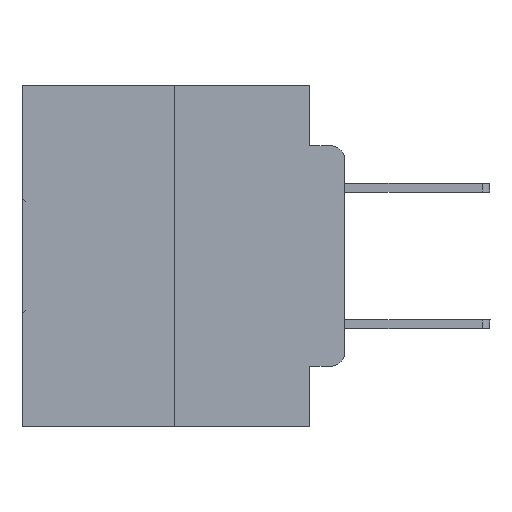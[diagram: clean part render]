
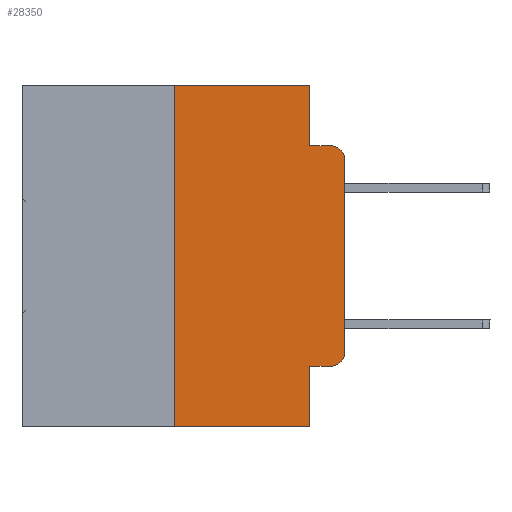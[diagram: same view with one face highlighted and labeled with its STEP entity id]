
A CAD part, left-side view. The second image highlights one B-rep face of the part: STEP entity #28350.
In plain terms, the highlighted planar face has unit normal (-1, 0, 0).
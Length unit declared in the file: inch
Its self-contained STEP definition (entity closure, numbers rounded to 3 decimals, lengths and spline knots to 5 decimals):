
#90 = CIRCLE ( 'NONE', #5570, 0.02 ) ;
#978 = CARTESIAN_POINT ( 'NONE',  ( 0., 0.25, 0. ) ) ;
#1286 = VECTOR ( 'NONE', #7229, 39.37008 ) ;
#1946 = CARTESIAN_POINT ( 'NONE',  ( 0., 0.25, -0.5 ) ) ;
#2361 = EDGE_CURVE ( 'NONE', #21545, #8161, #90, .T. ) ;
#2378 = VERTEX_POINT ( 'NONE', #16070 ) ;
#3023 = DIRECTION ( 'NONE',  ( -1., 0., 0. ) ) ;
#3044 = LINE ( 'NONE', #3188, #24980 ) ;
#3188 = CARTESIAN_POINT ( 'NONE',  ( 0., 0.25, 0. ) ) ;
#3230 = EDGE_CURVE ( 'NONE', #10841, #24574, #9522, .T. ) ;
#4170 = CARTESIAN_POINT ( 'NONE',  ( 0., 0.051, -0.0885 ) ) ;
#4710 = ORIENTED_EDGE ( 'NONE', *, *, #30780, .F. ) ;
#4950 = DIRECTION ( 'NONE',  ( 0., -1., 0. ) ) ;
#5284 = CARTESIAN_POINT ( 'NONE',  ( 0., 0.051, 0. ) ) ;
#5570 = AXIS2_PLACEMENT_3D ( 'NONE', #30448, #3023, #27502 ) ;
#5623 = CARTESIAN_POINT ( 'NONE',  ( 0., 0.473, 0. ) ) ;
#6782 = EDGE_CURVE ( 'NONE', #2378, #23884, #14330, .T. ) ;
#6934 = CARTESIAN_POINT ( 'NONE',  ( 0., 0.473, -0.5 ) ) ;
#7129 = CARTESIAN_POINT ( 'NONE',  ( 0., 0., 0. ) ) ;
#7229 = DIRECTION ( 'NONE',  ( 0., 0., 1. ) ) ;
#7676 = ORIENTED_EDGE ( 'NONE', *, *, #30650, .F. ) ;
#7956 = LINE ( 'NONE', #7129, #1286 ) ;
#8161 = VERTEX_POINT ( 'NONE', #27366 ) ;
#9522 = LINE ( 'NONE', #6934, #31732 ) ;
#9606 = CARTESIAN_POINT ( 'NONE',  ( 0., 0.051, -0.5 ) ) ;
#9624 = CARTESIAN_POINT ( 'NONE',  ( 0., 0.473, 0. ) ) ;
#10199 = ORIENTED_EDGE ( 'NONE', *, *, #25979, .F. ) ;
#10429 = AXIS2_PLACEMENT_3D ( 'NONE', #5623, #30745, #18219 ) ;
#10841 = VERTEX_POINT ( 'NONE', #1946 ) ;
#10940 = VECTOR ( 'NONE', #4950, 39.37008 ) ;
#11404 = CARTESIAN_POINT ( 'NONE',  ( 0., 0.02, -0.4115 ) ) ;
#12085 = DIRECTION ( 'NONE',  ( 0., 0., -1. ) ) ;
#12148 = DIRECTION ( 'NONE',  ( 0., -1., 0. ) ) ;
#12520 = EDGE_LOOP ( 'NONE', ( #16695, #15966, #7676, #10199, #21505, #4710, #30904, #24911, #22320, #30942 ) ) ;
#12539 = CARTESIAN_POINT ( 'NONE',  ( 0., 0.051, -0.0885 ) ) ;
#12789 = CARTESIAN_POINT ( 'NONE',  ( 0., 0., -0.3915 ) ) ;
#13038 = DIRECTION ( 'NONE',  ( 0., -1., 0. ) ) ;
#14039 = VECTOR ( 'NONE', #12148, 39.37008 ) ;
#14330 = LINE ( 'NONE', #30571, #24872 ) ;
#14619 = LINE ( 'NONE', #20100, #19346 ) ;
#15420 = VERTEX_POINT ( 'NONE', #978 ) ;
#15612 = PLANE ( 'NONE',  #10429 ) ;
#15622 = EDGE_CURVE ( 'NONE', #28118, #21545, #7956, .T. ) ;
#15966 = ORIENTED_EDGE ( 'NONE', *, *, #2361, .T. ) ;
#16070 = CARTESIAN_POINT ( 'NONE',  ( 0., 0.051, -0.4115 ) ) ;
#16695 = ORIENTED_EDGE ( 'NONE', *, *, #15622, .T. ) ;
#17127 = DIRECTION ( 'NONE',  ( 0., -1., 0. ) ) ;
#17555 = CIRCLE ( 'NONE', #30974, 0.02 ) ;
#18219 = DIRECTION ( 'NONE',  ( 0., 0., -1. ) ) ;
#19064 = DIRECTION ( 'NONE',  ( -1., 0., 0. ) ) ;
#19293 = DIRECTION ( 'NONE',  ( 0., 0., -1. ) ) ;
#19305 = CARTESIAN_POINT ( 'NONE',  ( 0., 0.051, 0. ) ) ;
#19346 = VECTOR ( 'NONE', #23236, 39.37008 ) ;
#20100 = CARTESIAN_POINT ( 'NONE',  ( 0., 0.051, 0. ) ) ;
#20176 = EDGE_CURVE ( 'NONE', #15420, #22908, #22264, .T. ) ;
#20800 = CARTESIAN_POINT ( 'NONE',  ( 0., 0., -0.1085 ) ) ;
#20823 = DIRECTION ( 'NONE',  ( 0., 0., 1. ) ) ;
#21505 = ORIENTED_EDGE ( 'NONE', *, *, #20176, .F. ) ;
#21545 = VERTEX_POINT ( 'NONE', #20800 ) ;
#22264 = LINE ( 'NONE', #9624, #14039 ) ;
#22320 = ORIENTED_EDGE ( 'NONE', *, *, #6782, .T. ) ;
#22908 = VERTEX_POINT ( 'NONE', #5284 ) ;
#23236 = DIRECTION ( 'NONE',  ( 0., 0., -1. ) ) ;
#23325 = VERTEX_POINT ( 'NONE', #4170 ) ;
#23841 = LINE ( 'NONE', #19305, #28900 ) ;
#23884 = VERTEX_POINT ( 'NONE', #11404 ) ;
#24367 = FACE_OUTER_BOUND ( 'NONE', #12520, .T. ) ;
#24574 = VERTEX_POINT ( 'NONE', #9606 ) ;
#24872 = VECTOR ( 'NONE', #13038, 39.37008 ) ;
#24911 = ORIENTED_EDGE ( 'NONE', *, *, #28251, .F. ) ;
#24980 = VECTOR ( 'NONE', #20823, 39.37008 ) ;
#25979 = EDGE_CURVE ( 'NONE', #22908, #23325, #23841, .T. ) ;
#27366 = CARTESIAN_POINT ( 'NONE',  ( 0., 0.02, -0.0885 ) ) ;
#27502 = DIRECTION ( 'NONE',  ( 0., 0., -1. ) ) ;
#28118 = VERTEX_POINT ( 'NONE', #12789 ) ;
#28251 = EDGE_CURVE ( 'NONE', #2378, #24574, #14619, .T. ) ;
#28350 = ADVANCED_FACE ( 'NONE', ( #24367 ), #15612, .F. ) ;
#28900 = VECTOR ( 'NONE', #12085, 39.37008 ) ;
#28968 = CARTESIAN_POINT ( 'NONE',  ( 0., 0.02, -0.3915 ) ) ;
#30412 = LINE ( 'NONE', #12539, #10940 ) ;
#30448 = CARTESIAN_POINT ( 'NONE',  ( 0., 0.02, -0.1085 ) ) ;
#30571 = CARTESIAN_POINT ( 'NONE',  ( 0., 0.051, -0.4115 ) ) ;
#30650 = EDGE_CURVE ( 'NONE', #23325, #8161, #30412, .T. ) ;
#30745 = DIRECTION ( 'NONE',  ( 1., 0., 0. ) ) ;
#30780 = EDGE_CURVE ( 'NONE', #10841, #15420, #3044, .T. ) ;
#30904 = ORIENTED_EDGE ( 'NONE', *, *, #3230, .T. ) ;
#30942 = ORIENTED_EDGE ( 'NONE', *, *, #31080, .T. ) ;
#30974 = AXIS2_PLACEMENT_3D ( 'NONE', #28968, #19064, #19293 ) ;
#31080 = EDGE_CURVE ( 'NONE', #23884, #28118, #17555, .T. ) ;
#31732 = VECTOR ( 'NONE', #17127, 39.37008 ) ;
